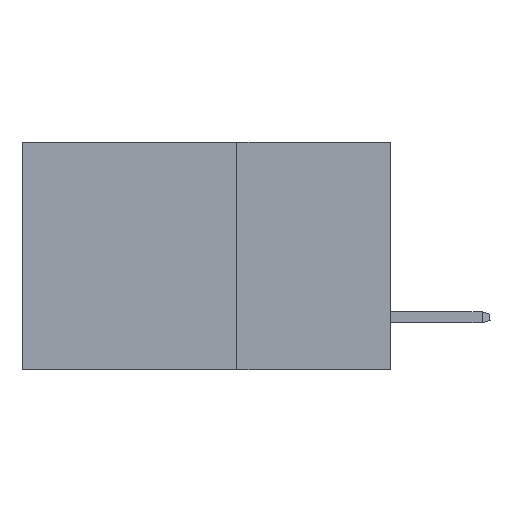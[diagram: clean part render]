
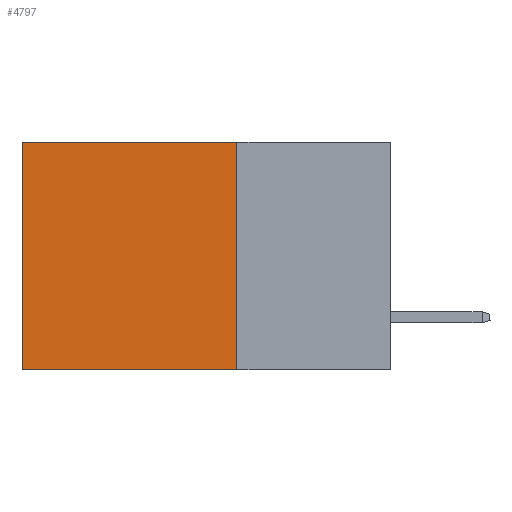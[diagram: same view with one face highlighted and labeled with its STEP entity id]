
A CAD part, left-side view. The second image highlights one B-rep face of the part: STEP entity #4797.
In plain terms, the highlighted planar face has unit normal (-1, 0, 0).
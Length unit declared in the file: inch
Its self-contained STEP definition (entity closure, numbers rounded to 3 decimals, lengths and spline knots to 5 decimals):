
#482 = CARTESIAN_POINT ( 'NONE',  ( 0.2875, 0.25, 0. ) ) ;
#748 = ORIENTED_EDGE ( 'NONE', *, *, #16519, .F. ) ;
#1594 = VECTOR ( 'NONE', #1879, 39.37008 ) ;
#1879 = DIRECTION ( 'NONE',  ( 0., 1., 0. ) ) ;
#1915 = PLANE ( 'NONE',  #12498 ) ;
#1955 = CARTESIAN_POINT ( 'NONE',  ( 0.2875, 0.25, 0. ) ) ;
#2014 = ORIENTED_EDGE ( 'NONE', *, *, #2992, .T. ) ;
#2359 = VECTOR ( 'NONE', #14989, 39.37008 ) ;
#2800 = CARTESIAN_POINT ( 'NONE',  ( 0.2875, 0.25, -0.37 ) ) ;
#2992 = EDGE_CURVE ( 'NONE', #5811, #5851, #17355, .T. ) ;
#4611 = CARTESIAN_POINT ( 'NONE',  ( 0.2875, 0.25, 0. ) ) ;
#4760 = CARTESIAN_POINT ( 'NONE',  ( 0.2875, 0.6, -0.37 ) ) ;
#4797 = ADVANCED_FACE ( 'NONE', ( #15963 ), #1915, .F. ) ;
#5811 = VERTEX_POINT ( 'NONE', #9796 ) ;
#5841 = EDGE_LOOP ( 'NONE', ( #10649, #9066, #748, #2014 ) ) ;
#5851 = VERTEX_POINT ( 'NONE', #6947 ) ;
#6775 = VECTOR ( 'NONE', #16736, 39.37008 ) ;
#6947 = CARTESIAN_POINT ( 'NONE',  ( 0.2875, 0.6, 0. ) ) ;
#7701 = VECTOR ( 'NONE', #17298, 39.37008 ) ;
#7714 = EDGE_CURVE ( 'NONE', #5851, #15198, #16247, .T. ) ;
#8405 = LINE ( 'NONE', #1955, #2359 ) ;
#9066 = ORIENTED_EDGE ( 'NONE', *, *, #9073, .F. ) ;
#9073 = EDGE_CURVE ( 'NONE', #16958, #15198, #10592, .T. ) ;
#9796 = CARTESIAN_POINT ( 'NONE',  ( 0.2875, 0.25, 0. ) ) ;
#9984 = CARTESIAN_POINT ( 'NONE',  ( 0.2875, 0.6, 0. ) ) ;
#10592 = LINE ( 'NONE', #13594, #6775 ) ;
#10649 = ORIENTED_EDGE ( 'NONE', *, *, #7714, .T. ) ;
#12498 = AXIS2_PLACEMENT_3D ( 'NONE', #4611, #14822, #13367 ) ;
#13367 = DIRECTION ( 'NONE',  ( 0., 0., -1. ) ) ;
#13594 = CARTESIAN_POINT ( 'NONE',  ( 0.2875, 0.25, -0.37 ) ) ;
#14822 = DIRECTION ( 'NONE',  ( 1., 0., 0. ) ) ;
#14989 = DIRECTION ( 'NONE',  ( 0., 0., -1. ) ) ;
#15198 = VERTEX_POINT ( 'NONE', #4760 ) ;
#15963 = FACE_OUTER_BOUND ( 'NONE', #5841, .T. ) ;
#16247 = LINE ( 'NONE', #9984, #7701 ) ;
#16519 = EDGE_CURVE ( 'NONE', #5811, #16958, #8405, .T. ) ;
#16736 = DIRECTION ( 'NONE',  ( 0., 1., 0. ) ) ;
#16958 = VERTEX_POINT ( 'NONE', #2800 ) ;
#17298 = DIRECTION ( 'NONE',  ( 0., 0., -1. ) ) ;
#17355 = LINE ( 'NONE', #482, #1594 ) ;
